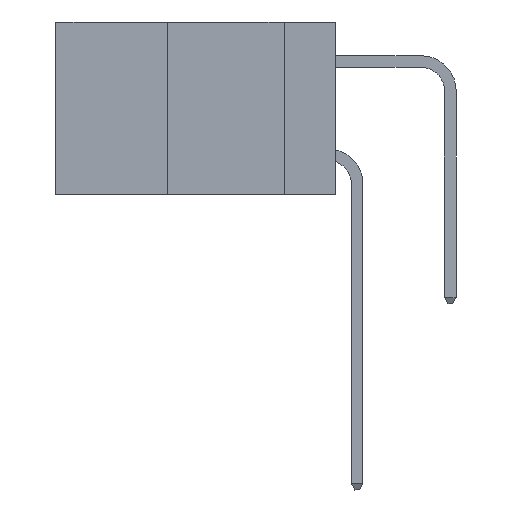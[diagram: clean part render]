
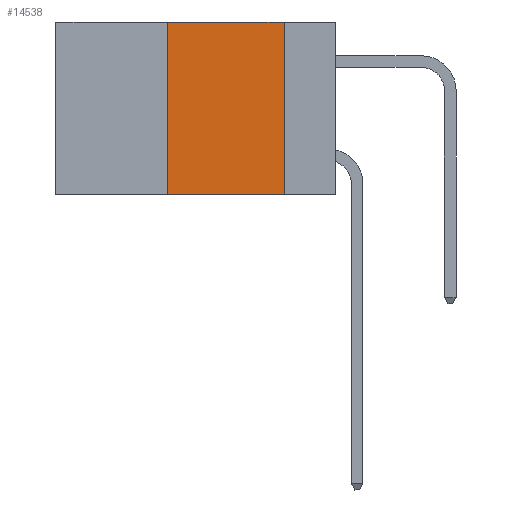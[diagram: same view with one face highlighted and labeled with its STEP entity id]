
A CAD part, left-side view. The second image highlights one B-rep face of the part: STEP entity #14538.
In plain terms, the highlighted planar face has unit normal (-1, 0, 0).
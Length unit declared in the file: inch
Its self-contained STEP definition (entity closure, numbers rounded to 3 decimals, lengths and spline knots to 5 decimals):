
#1001 = VECTOR ( 'NONE', #17438, 39.37008 ) ;
#1592 = VECTOR ( 'NONE', #12801, 39.37008 ) ;
#2224 = LINE ( 'NONE', #18420, #1592 ) ;
#2649 = VERTEX_POINT ( 'NONE', #24355 ) ;
#2766 = CARTESIAN_POINT ( 'NONE',  ( 0., 0.11, 0. ) ) ;
#2951 = VECTOR ( 'NONE', #8805, 39.37008 ) ;
#4015 = CARTESIAN_POINT ( 'NONE',  ( 0., 0.11, 0. ) ) ;
#4107 = VERTEX_POINT ( 'NONE', #2766 ) ;
#4258 = CARTESIAN_POINT ( 'NONE',  ( 0., 0.6, 0. ) ) ;
#4315 = VECTOR ( 'NONE', #6229, 39.37008 ) ;
#4918 = LINE ( 'NONE', #4258, #4315 ) ;
#5962 = CARTESIAN_POINT ( 'NONE',  ( 0., 0.6, 0. ) ) ;
#6229 = DIRECTION ( 'NONE',  ( 0., -1., 0. ) ) ;
#7958 = DIRECTION ( 'NONE',  ( 1., 0., 0. ) ) ;
#8172 = LINE ( 'NONE', #14481, #2951 ) ;
#8470 = ORIENTED_EDGE ( 'NONE', *, *, #10127, .F. ) ;
#8805 = DIRECTION ( 'NONE',  ( 0., -1., 0. ) ) ;
#10127 = EDGE_CURVE ( 'NONE', #16596, #14171, #2224, .T. ) ;
#10416 = CARTESIAN_POINT ( 'NONE',  ( 0., 0.36, 0. ) ) ;
#10496 = AXIS2_PLACEMENT_3D ( 'NONE', #5962, #7958, #21234 ) ;
#12801 = DIRECTION ( 'NONE',  ( 0., 0., 1. ) ) ;
#13953 = EDGE_CURVE ( 'NONE', #4107, #2649, #20845, .T. ) ;
#14149 = ORIENTED_EDGE ( 'NONE', *, *, #19214, .T. ) ;
#14171 = VERTEX_POINT ( 'NONE', #10416 ) ;
#14481 = CARTESIAN_POINT ( 'NONE',  ( 0., 0.6, -0.37 ) ) ;
#14538 = ADVANCED_FACE ( 'NONE', ( #23174 ), #17419, .F. ) ;
#15971 = EDGE_CURVE ( 'NONE', #14171, #4107, #4918, .T. ) ;
#16596 = VERTEX_POINT ( 'NONE', #23462 ) ;
#17419 = PLANE ( 'NONE',  #10496 ) ;
#17429 = EDGE_LOOP ( 'NONE', ( #24412, #20647, #8470, #14149 ) ) ;
#17438 = DIRECTION ( 'NONE',  ( 0., 0., -1. ) ) ;
#18420 = CARTESIAN_POINT ( 'NONE',  ( 0., 0.36, 0. ) ) ;
#19214 = EDGE_CURVE ( 'NONE', #16596, #2649, #8172, .T. ) ;
#20647 = ORIENTED_EDGE ( 'NONE', *, *, #15971, .F. ) ;
#20845 = LINE ( 'NONE', #4015, #1001 ) ;
#21234 = DIRECTION ( 'NONE',  ( 0., 0., -1. ) ) ;
#23174 = FACE_OUTER_BOUND ( 'NONE', #17429, .T. ) ;
#23462 = CARTESIAN_POINT ( 'NONE',  ( 0., 0.36, -0.37 ) ) ;
#24355 = CARTESIAN_POINT ( 'NONE',  ( 0., 0.11, -0.37 ) ) ;
#24412 = ORIENTED_EDGE ( 'NONE', *, *, #13953, .F. ) ;
